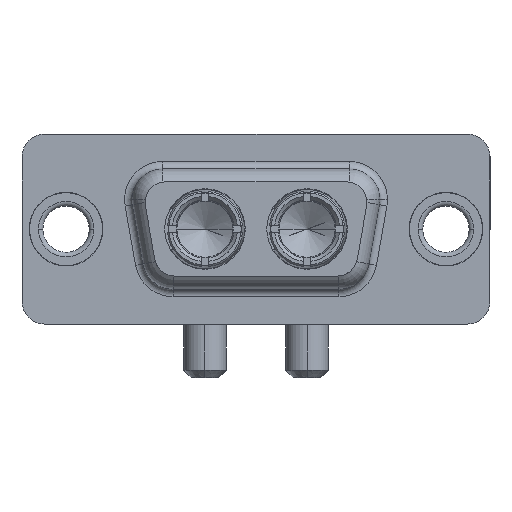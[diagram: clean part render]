
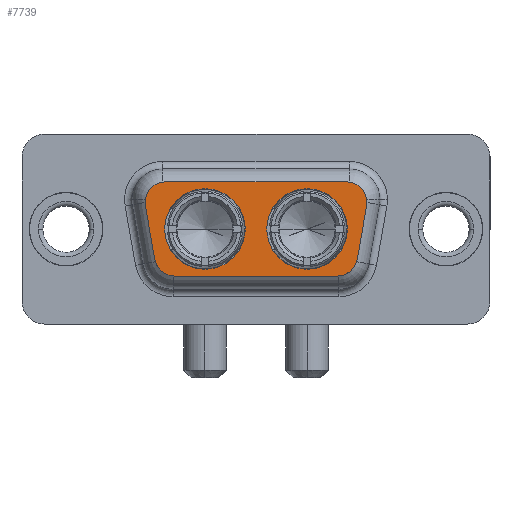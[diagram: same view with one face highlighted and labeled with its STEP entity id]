
A CAD part, top view. The second image highlights one B-rep face of the part: STEP entity #7739.
In plain terms, the highlighted planar face has unit normal (0, 0, 1).
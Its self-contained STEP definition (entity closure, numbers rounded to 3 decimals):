
#166 = AXIS2_PLACEMENT_3D ( 'NONE', #1122, #2525, #8310 ) ;
#275 = VERTEX_POINT ( 'NONE', #6835 ) ;
#343 = EDGE_CURVE ( 'NONE', #4115, #776, #1070, .T. ) ;
#366 = VERTEX_POINT ( 'NONE', #2261 ) ;
#714 = CARTESIAN_POINT ( 'NONE',  ( 13.21, 0., 6.2 ) ) ;
#776 = VERTEX_POINT ( 'NONE', #6928 ) ;
#1070 = CIRCLE ( 'NONE', #9773, 1.35 ) ;
#1080 = EDGE_CURVE ( 'NONE', #275, #366, #4382, .T. ) ;
#1122 = CARTESIAN_POINT ( 'NONE',  ( 6.55, 1.75, 6.2 ) ) ;
#1199 = CARTESIAN_POINT ( 'NONE',  ( 6.55, 3.1, 6.2 ) ) ;
#1247 = CARTESIAN_POINT ( 'NONE',  ( 7.167, -1.75, 6.2 ) ) ;
#1422 = CARTESIAN_POINT ( 'NONE',  ( 7.167, -3.1, 6.2 ) ) ;
#1428 = FACE_OUTER_BOUND ( 'NONE', #10280, .T. ) ;
#1469 = DIRECTION ( 'NONE',  ( 1., 0., 0. ) ) ;
#1478 = DIRECTION ( 'NONE',  ( -1., 0., 0. ) ) ;
#1583 = ORIENTED_EDGE ( 'NONE', *, *, #9204, .T. ) ;
#1617 = AXIS2_PLACEMENT_3D ( 'NONE', #1247, #6856, #6092 ) ;
#1935 = EDGE_CURVE ( 'NONE', #4877, #2124, #6951, .T. ) ;
#1968 = DIRECTION ( 'NONE',  ( 1., 0., 0. ) ) ;
#2031 = DIRECTION ( 'NONE',  ( 0., 0., 1. ) ) ;
#2092 = AXIS2_PLACEMENT_3D ( 'NONE', #9788, #7536, #5039 ) ;
#2124 = VERTEX_POINT ( 'NONE', #6942 ) ;
#2127 = DIRECTION ( 'NONE',  ( 0., 0., 1. ) ) ;
#2261 = CARTESIAN_POINT ( 'NONE',  ( 6.55, 3.1, 6.2 ) ) ;
#2453 = EDGE_CURVE ( 'NONE', #776, #4707, #4489, .T. ) ;
#2464 = VERTEX_POINT ( 'NONE', #3568 ) ;
#2512 = CARTESIAN_POINT ( 'NONE',  ( 17.833, -3.1, 6.2 ) ) ;
#2525 = DIRECTION ( 'NONE',  ( 0., 0., 1. ) ) ;
#2885 = DIRECTION ( 'NONE',  ( -1., 0., 0. ) ) ;
#2889 = AXIS2_PLACEMENT_3D ( 'NONE', #4062, #7415, #8197 ) ;
#2966 = CIRCLE ( 'NONE', #3137, 1.35 ) ;
#3022 = ORIENTED_EDGE ( 'NONE', *, *, #343, .T. ) ;
#3137 = AXIS2_PLACEMENT_3D ( 'NONE', #3664, #2031, #7701 ) ;
#3218 = CARTESIAN_POINT ( 'NONE',  ( 6.49, 0., 6.2 ) ) ;
#3376 = EDGE_CURVE ( 'NONE', #366, #9987, #2966, .T. ) ;
#3404 = ORIENTED_EDGE ( 'NONE', *, *, #7085, .F. ) ;
#3411 = VECTOR ( 'NONE', #4434, 1000. ) ;
#3568 = CARTESIAN_POINT ( 'NONE',  ( 11.79, 0., 6.2 ) ) ;
#3642 = EDGE_LOOP ( 'NONE', ( #8996, #9100 ) ) ;
#3664 = CARTESIAN_POINT ( 'NONE',  ( 6.55, 1.75, 6.2 ) ) ;
#3978 = CIRCLE ( 'NONE', #1617, 1.35 ) ;
#4062 = CARTESIAN_POINT ( 'NONE',  ( 9.14, 0., 6.2 ) ) ;
#4115 = VERTEX_POINT ( 'NONE', #5271 ) ;
#4122 = LINE ( 'NONE', #2512, #9601 ) ;
#4382 = LINE ( 'NONE', #1199, #3411 ) ;
#4434 = DIRECTION ( 'NONE',  ( -1., 0., 0. ) ) ;
#4489 = LINE ( 'NONE', #5164, #8823 ) ;
#4574 = CARTESIAN_POINT ( 'NONE',  ( 9.14, 0., 6.2 ) ) ;
#4659 = PLANE ( 'NONE',  #6584 ) ;
#4680 = LINE ( 'NONE', #7647, #9850 ) ;
#4707 = VERTEX_POINT ( 'NONE', #5456 ) ;
#4717 = EDGE_CURVE ( 'NONE', #6715, #8494, #4680, .T. ) ;
#4721 = CARTESIAN_POINT ( 'NONE',  ( 5.838, -1.984, 6.2 ) ) ;
#4877 = VERTEX_POINT ( 'NONE', #714 ) ;
#4989 = ORIENTED_EDGE ( 'NONE', *, *, #7829, .T. ) ;
#5010 = AXIS2_PLACEMENT_3D ( 'NONE', #6003, #8509, #2885 ) ;
#5039 = DIRECTION ( 'NONE',  ( 1., 0., 0. ) ) ;
#5159 = ORIENTED_EDGE ( 'NONE', *, *, #2453, .T. ) ;
#5164 = CARTESIAN_POINT ( 'NONE',  ( 19.779, 1.516, 6.2 ) ) ;
#5220 = DIRECTION ( 'NONE',  ( 0.174, 0.985, 0. ) ) ;
#5271 = CARTESIAN_POINT ( 'NONE',  ( 17.833, -3.1, 6.2 ) ) ;
#5405 = ORIENTED_EDGE ( 'NONE', *, *, #3376, .T. ) ;
#5456 = CARTESIAN_POINT ( 'NONE',  ( 19.779, 1.516, 6.2 ) ) ;
#5525 = CIRCLE ( 'NONE', #8356, 2.65 ) ;
#5531 = EDGE_LOOP ( 'NONE', ( #5551, #3404 ) ) ;
#5551 = ORIENTED_EDGE ( 'NONE', *, *, #7788, .F. ) ;
#5581 = VERTEX_POINT ( 'NONE', #1422 ) ;
#5665 = ORIENTED_EDGE ( 'NONE', *, *, #1080, .T. ) ;
#5741 = DIRECTION ( 'NONE',  ( 1., 0., 0. ) ) ;
#6003 = CARTESIAN_POINT ( 'NONE',  ( 18.45, 1.75, 6.2 ) ) ;
#6092 = DIRECTION ( 'NONE',  ( -1., 0., 0. ) ) ;
#6169 = CARTESIAN_POINT ( 'NONE',  ( 17.833, -1.75, 6.2 ) ) ;
#6217 = FACE_BOUND ( 'NONE', #3642, .T. ) ;
#6481 = VERTEX_POINT ( 'NONE', #3218 ) ;
#6534 = ORIENTED_EDGE ( 'NONE', *, *, #4717, .T. ) ;
#6547 = EDGE_CURVE ( 'NONE', #9987, #6715, #9548, .T. ) ;
#6584 = AXIS2_PLACEMENT_3D ( 'NONE', #9460, #8672, #1478 ) ;
#6715 = VERTEX_POINT ( 'NONE', #8566 ) ;
#6835 = CARTESIAN_POINT ( 'NONE',  ( 18.45, 3.1, 6.2 ) ) ;
#6856 = DIRECTION ( 'NONE',  ( 0., 0., 1. ) ) ;
#6928 = CARTESIAN_POINT ( 'NONE',  ( 19.162, -1.984, 6.2 ) ) ;
#6942 = CARTESIAN_POINT ( 'NONE',  ( 18.51, 0., 6.2 ) ) ;
#6951 = CIRCLE ( 'NONE', #2092, 2.65 ) ;
#7085 = EDGE_CURVE ( 'NONE', #6481, #2464, #8582, .T. ) ;
#7107 = ORIENTED_EDGE ( 'NONE', *, *, #9651, .T. ) ;
#7413 = AXIS2_PLACEMENT_3D ( 'NONE', #4574, #2127, #1968 ) ;
#7415 = DIRECTION ( 'NONE',  ( 0., 0., 1. ) ) ;
#7536 = DIRECTION ( 'NONE',  ( 0., 0., 1. ) ) ;
#7647 = CARTESIAN_POINT ( 'NONE',  ( 5.838, -1.984, 6.2 ) ) ;
#7701 = DIRECTION ( 'NONE',  ( 1., 0., 0. ) ) ;
#7719 = DIRECTION ( 'NONE',  ( 0., 0., 1. ) ) ;
#7739 = ADVANCED_FACE ( 'NONE', ( #6217, #10238, #1428 ), #4659, .F. ) ;
#7788 = EDGE_CURVE ( 'NONE', #2464, #6481, #9433, .T. ) ;
#7829 = EDGE_CURVE ( 'NONE', #5581, #4115, #4122, .T. ) ;
#7844 = DIRECTION ( 'NONE',  ( 0.174, -0.985, 0. ) ) ;
#7858 = ORIENTED_EDGE ( 'NONE', *, *, #6547, .T. ) ;
#8058 = CARTESIAN_POINT ( 'NONE',  ( 5.2, 1.75, 6.2 ) ) ;
#8172 = DIRECTION ( 'NONE',  ( -1., 0., 0. ) ) ;
#8197 = DIRECTION ( 'NONE',  ( 1., 0., 0. ) ) ;
#8310 = DIRECTION ( 'NONE',  ( 1., 0., 0. ) ) ;
#8356 = AXIS2_PLACEMENT_3D ( 'NONE', #10336, #7719, #1469 ) ;
#8494 = VERTEX_POINT ( 'NONE', #4721 ) ;
#8509 = DIRECTION ( 'NONE',  ( 0., 0., 1. ) ) ;
#8566 = CARTESIAN_POINT ( 'NONE',  ( 5.221, 1.516, 6.2 ) ) ;
#8582 = CIRCLE ( 'NONE', #7413, 2.65 ) ;
#8672 = DIRECTION ( 'NONE',  ( 0., 0., -1. ) ) ;
#8823 = VECTOR ( 'NONE', #5220, 1000. ) ;
#8996 = ORIENTED_EDGE ( 'NONE', *, *, #9371, .F. ) ;
#9100 = ORIENTED_EDGE ( 'NONE', *, *, #1935, .F. ) ;
#9204 = EDGE_CURVE ( 'NONE', #4707, #275, #10022, .T. ) ;
#9365 = DIRECTION ( 'NONE',  ( 0., 0., 1. ) ) ;
#9371 = EDGE_CURVE ( 'NONE', #2124, #4877, #5525, .T. ) ;
#9433 = CIRCLE ( 'NONE', #2889, 2.65 ) ;
#9460 = CARTESIAN_POINT ( 'NONE',  ( 7.167, -1.75, 6.2 ) ) ;
#9548 = CIRCLE ( 'NONE', #166, 1.35 ) ;
#9601 = VECTOR ( 'NONE', #5741, 1000. ) ;
#9651 = EDGE_CURVE ( 'NONE', #8494, #5581, #3978, .T. ) ;
#9773 = AXIS2_PLACEMENT_3D ( 'NONE', #6169, #9365, #8172 ) ;
#9788 = CARTESIAN_POINT ( 'NONE',  ( 15.86, 0., 6.2 ) ) ;
#9850 = VECTOR ( 'NONE', #7844, 1000. ) ;
#9987 = VERTEX_POINT ( 'NONE', #8058 ) ;
#10022 = CIRCLE ( 'NONE', #5010, 1.35 ) ;
#10238 = FACE_BOUND ( 'NONE', #5531, .T. ) ;
#10280 = EDGE_LOOP ( 'NONE', ( #7107, #4989, #3022, #5159, #1583, #5665, #5405, #7858, #6534 ) ) ;
#10336 = CARTESIAN_POINT ( 'NONE',  ( 15.86, 0., 6.2 ) ) ;
